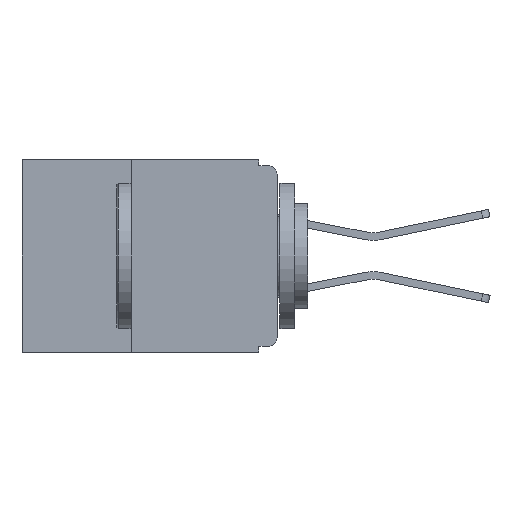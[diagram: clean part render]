
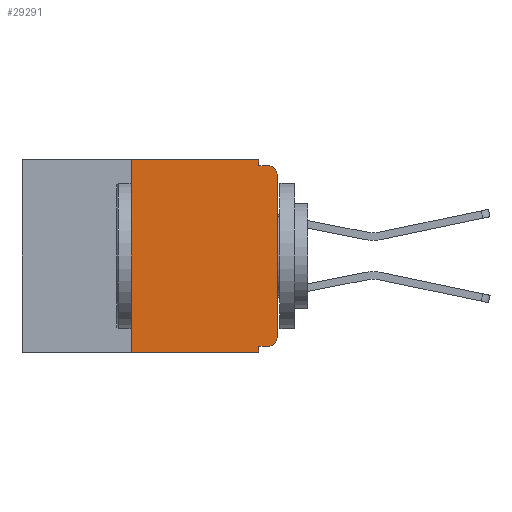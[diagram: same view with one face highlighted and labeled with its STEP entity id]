
A CAD part, left-side view. The second image highlights one B-rep face of the part: STEP entity #29291.
In plain terms, the highlighted planar face has unit normal (-1, 0, 0).
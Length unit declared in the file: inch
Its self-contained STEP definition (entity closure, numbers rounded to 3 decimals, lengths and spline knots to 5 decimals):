
#69 = CARTESIAN_POINT ( 'NONE',  ( 0., 0.031, 0. ) ) ;
#250 = DIRECTION ( 'NONE',  ( 0., 0., 1. ) ) ;
#533 = DIRECTION ( 'NONE',  ( 0., 0., -1. ) ) ;
#767 = CARTESIAN_POINT ( 'NONE',  ( 0., 0.25, -0.33 ) ) ;
#1053 = CARTESIAN_POINT ( 'NONE',  ( 0., 0., -0.025 ) ) ;
#1190 = DIRECTION ( 'NONE',  ( 0., 0., -1. ) ) ;
#1370 = VECTOR ( 'NONE', #10776, 39.37008 ) ;
#1375 = VECTOR ( 'NONE', #3914, 39.37008 ) ;
#2106 = CARTESIAN_POINT ( 'NONE',  ( 0., 0., -0.305 ) ) ;
#3179 = LINE ( 'NONE', #30017, #1370 ) ;
#3257 = ORIENTED_EDGE ( 'NONE', *, *, #11253, .T. ) ;
#3914 = DIRECTION ( 'NONE',  ( 0., 0., 1. ) ) ;
#3931 = ORIENTED_EDGE ( 'NONE', *, *, #28845, .T. ) ;
#4038 = ORIENTED_EDGE ( 'NONE', *, *, #16723, .F. ) ;
#4808 = ORIENTED_EDGE ( 'NONE', *, *, #31192, .F. ) ;
#5259 = AXIS2_PLACEMENT_3D ( 'NONE', #34412, #18086, #1190 ) ;
#5426 = ORIENTED_EDGE ( 'NONE', *, *, #23227, .F. ) ;
#5448 = LINE ( 'NONE', #17177, #26687 ) ;
#5524 = ORIENTED_EDGE ( 'NONE', *, *, #17767, .F. ) ;
#5981 = VERTEX_POINT ( 'NONE', #767 ) ;
#6188 = ORIENTED_EDGE ( 'NONE', *, *, #29383, .T. ) ;
#6282 = EDGE_CURVE ( 'NONE', #18663, #33398, #31548, .T. ) ;
#6338 = ORIENTED_EDGE ( 'NONE', *, *, #26917, .F. ) ;
#6462 = DIRECTION ( 'NONE',  ( 0., 0., -1. ) ) ;
#6771 = ORIENTED_EDGE ( 'NONE', *, *, #6282, .F. ) ;
#6870 = ORIENTED_EDGE ( 'NONE', *, *, #11667, .T. ) ;
#6976 = CARTESIAN_POINT ( 'NONE',  ( 0., 0.031, -0.33 ) ) ;
#7474 = PLANE ( 'NONE',  #13758 ) ;
#8861 = DIRECTION ( 'NONE',  ( 0., -1., 0. ) ) ;
#8987 = LINE ( 'NONE', #12318, #1375 ) ;
#9605 = VECTOR ( 'NONE', #22054, 39.37008 ) ;
#10413 = DIRECTION ( 'NONE',  ( 0., 0., -1. ) ) ;
#10776 = DIRECTION ( 'NONE',  ( 0., -1., 0. ) ) ;
#11253 = EDGE_CURVE ( 'NONE', #23078, #21682, #8987, .T. ) ;
#11409 = VERTEX_POINT ( 'NONE', #34949 ) ;
#11667 = EDGE_CURVE ( 'NONE', #18663, #23078, #32623, .T. ) ;
#12253 = EDGE_LOOP ( 'NONE', ( #3257, #3931, #4038, #4808, #5426, #5524, #6188, #6338, #6771, #6870 ) ) ;
#12318 = CARTESIAN_POINT ( 'NONE',  ( 0., 0., 0. ) ) ;
#12493 = FACE_OUTER_BOUND ( 'NONE', #12253, .T. ) ;
#13132 = CARTESIAN_POINT ( 'NONE',  ( 0., 0.031, 0. ) ) ;
#13645 = CARTESIAN_POINT ( 'NONE',  ( 0., 0.015, -0.01 ) ) ;
#13758 = AXIS2_PLACEMENT_3D ( 'NONE', #18715, #26926, #10413 ) ;
#14662 = CARTESIAN_POINT ( 'NONE',  ( 0., 0., -0.01 ) ) ;
#16723 = EDGE_CURVE ( 'NONE', #19930, #30660, #31895, .T. ) ;
#17177 = CARTESIAN_POINT ( 'NONE',  ( 0., 0.25, -0.33 ) ) ;
#17390 = VECTOR ( 'NONE', #17449, 39.37008 ) ;
#17449 = DIRECTION ( 'NONE',  ( 0., -1., 0. ) ) ;
#17457 = DIRECTION ( 'NONE',  ( -1., 0., 0. ) ) ;
#17767 = EDGE_CURVE ( 'NONE', #5981, #11409, #5448, .T. ) ;
#18086 = DIRECTION ( 'NONE',  ( -1., 0., 0. ) ) ;
#18663 = VERTEX_POINT ( 'NONE', #32396 ) ;
#18715 = CARTESIAN_POINT ( 'NONE',  ( 0., 0.437, 0. ) ) ;
#19151 = VECTOR ( 'NONE', #8861, 39.37008 ) ;
#19752 = VECTOR ( 'NONE', #29547, 39.37008 ) ;
#19930 = VERTEX_POINT ( 'NONE', #26950 ) ;
#20475 = CARTESIAN_POINT ( 'NONE',  ( 0., 0.031, -0.33 ) ) ;
#21131 = VERTEX_POINT ( 'NONE', #6976 ) ;
#21682 = VERTEX_POINT ( 'NONE', #1053 ) ;
#21715 = CARTESIAN_POINT ( 'NONE',  ( 0., 0.031, -0.32 ) ) ;
#22054 = DIRECTION ( 'NONE',  ( 0., 1., 0. ) ) ;
#22280 = CARTESIAN_POINT ( 'NONE',  ( 0., 0., -0.32 ) ) ;
#22372 = AXIS2_PLACEMENT_3D ( 'NONE', #33762, #17457, #533 ) ;
#23078 = VERTEX_POINT ( 'NONE', #2106 ) ;
#23227 = EDGE_CURVE ( 'NONE', #11409, #29529, #26365, .T. ) ;
#25498 = VECTOR ( 'NONE', #6462, 39.37008 ) ;
#26365 = LINE ( 'NONE', #28165, #19151 ) ;
#26372 = LINE ( 'NONE', #20475, #25498 ) ;
#26687 = VECTOR ( 'NONE', #250, 39.37008 ) ;
#26917 = EDGE_CURVE ( 'NONE', #33398, #21131, #26372, .T. ) ;
#26926 = DIRECTION ( 'NONE',  ( 1., 0., 0. ) ) ;
#26950 = CARTESIAN_POINT ( 'NONE',  ( 0., 0.031, -0.01 ) ) ;
#28165 = CARTESIAN_POINT ( 'NONE',  ( 0., 0.437, 0. ) ) ;
#28845 = EDGE_CURVE ( 'NONE', #21682, #30660, #34740, .T. ) ;
#29291 = ADVANCED_FACE ( 'NONE', ( #12493 ), #7474, .F. ) ;
#29383 = EDGE_CURVE ( 'NONE', #5981, #21131, #3179, .T. ) ;
#29529 = VERTEX_POINT ( 'NONE', #69 ) ;
#29547 = DIRECTION ( 'NONE',  ( 0., 0., -1. ) ) ;
#30017 = CARTESIAN_POINT ( 'NONE',  ( 0., 0.437, -0.33 ) ) ;
#30660 = VERTEX_POINT ( 'NONE', #13645 ) ;
#31192 = EDGE_CURVE ( 'NONE', #29529, #19930, #34200, .T. ) ;
#31548 = LINE ( 'NONE', #22280, #9605 ) ;
#31895 = LINE ( 'NONE', #14662, #17390 ) ;
#32396 = CARTESIAN_POINT ( 'NONE',  ( 0., 0.015, -0.32 ) ) ;
#32623 = CIRCLE ( 'NONE', #22372, 0.015 ) ;
#33398 = VERTEX_POINT ( 'NONE', #21715 ) ;
#33762 = CARTESIAN_POINT ( 'NONE',  ( 0., 0.015, -0.305 ) ) ;
#34200 = LINE ( 'NONE', #13132, #19752 ) ;
#34412 = CARTESIAN_POINT ( 'NONE',  ( 0., 0.015, -0.025 ) ) ;
#34740 = CIRCLE ( 'NONE', #5259, 0.015 ) ;
#34949 = CARTESIAN_POINT ( 'NONE',  ( 0., 0.25, 0. ) ) ;
